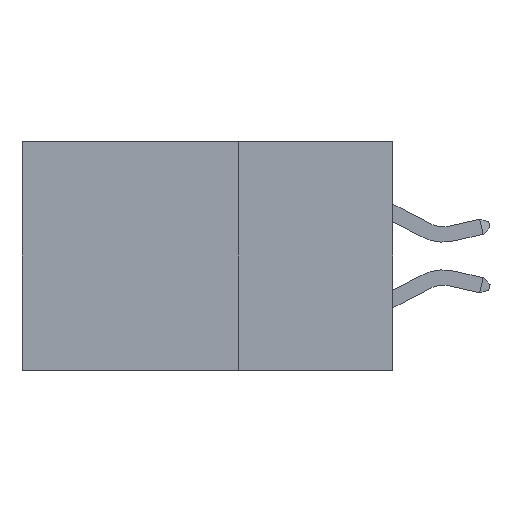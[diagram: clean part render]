
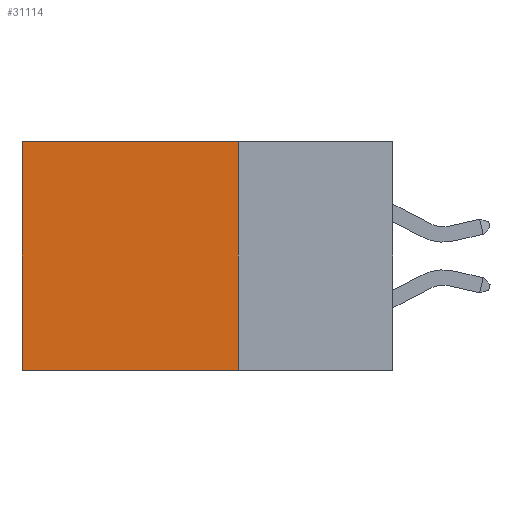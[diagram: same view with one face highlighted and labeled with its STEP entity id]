
A CAD part, left-side view. The second image highlights one B-rep face of the part: STEP entity #31114.
In plain terms, the highlighted planar face has unit normal (-1, 0, 0).
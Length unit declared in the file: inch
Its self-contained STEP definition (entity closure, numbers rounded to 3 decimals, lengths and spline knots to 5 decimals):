
#71 = LINE ( 'NONE', #34770, #13173 ) ;
#74 = CARTESIAN_POINT ( 'NONE',  ( 0.2875, 0.25, -0.37 ) ) ;
#258 = AXIS2_PLACEMENT_3D ( 'NONE', #278, #2641, #8161 ) ;
#278 = CARTESIAN_POINT ( 'NONE',  ( 0.2875, 0.25, 0. ) ) ;
#772 = CARTESIAN_POINT ( 'NONE',  ( 0.2875, 0.6, 0. ) ) ;
#2343 = CARTESIAN_POINT ( 'NONE',  ( 0.2875, 0.25, 0. ) ) ;
#2641 = DIRECTION ( 'NONE',  ( 1., 0., 0. ) ) ;
#3703 = ORIENTED_EDGE ( 'NONE', *, *, #32544, .F. ) ;
#3853 = EDGE_CURVE ( 'NONE', #13371, #12903, #31158, .T. ) ;
#4574 = DIRECTION ( 'NONE',  ( 0., 1., 0. ) ) ;
#4733 = FACE_OUTER_BOUND ( 'NONE', #22316, .T. ) ;
#5043 = LINE ( 'NONE', #17857, #17332 ) ;
#5070 = VECTOR ( 'NONE', #13770, 39.37008 ) ;
#7614 = VERTEX_POINT ( 'NONE', #25218 ) ;
#8161 = DIRECTION ( 'NONE',  ( 0., 0., -1. ) ) ;
#10586 = EDGE_CURVE ( 'NONE', #13371, #14467, #5043, .T. ) ;
#12903 = VERTEX_POINT ( 'NONE', #19934 ) ;
#13173 = VECTOR ( 'NONE', #33191, 39.37008 ) ;
#13371 = VERTEX_POINT ( 'NONE', #33732 ) ;
#13546 = DIRECTION ( 'NONE',  ( 0., 0., -1. ) ) ;
#13610 = ORIENTED_EDGE ( 'NONE', *, *, #18839, .T. ) ;
#13770 = DIRECTION ( 'NONE',  ( 0., 1., 0. ) ) ;
#14467 = VERTEX_POINT ( 'NONE', #772 ) ;
#15407 = ORIENTED_EDGE ( 'NONE', *, *, #10586, .T. ) ;
#16140 = PLANE ( 'NONE',  #258 ) ;
#17332 = VECTOR ( 'NONE', #4574, 39.37008 ) ;
#17857 = CARTESIAN_POINT ( 'NONE',  ( 0.2875, 0.25, 0. ) ) ;
#18105 = ORIENTED_EDGE ( 'NONE', *, *, #3853, .F. ) ;
#18839 = EDGE_CURVE ( 'NONE', #14467, #7614, #71, .T. ) ;
#19503 = LINE ( 'NONE', #74, #5070 ) ;
#19934 = CARTESIAN_POINT ( 'NONE',  ( 0.2875, 0.25, -0.37 ) ) ;
#22316 = EDGE_LOOP ( 'NONE', ( #13610, #3703, #18105, #15407 ) ) ;
#25218 = CARTESIAN_POINT ( 'NONE',  ( 0.2875, 0.6, -0.37 ) ) ;
#26887 = VECTOR ( 'NONE', #13546, 39.37008 ) ;
#31114 = ADVANCED_FACE ( 'NONE', ( #4733 ), #16140, .F. ) ;
#31158 = LINE ( 'NONE', #2343, #26887 ) ;
#32544 = EDGE_CURVE ( 'NONE', #12903, #7614, #19503, .T. ) ;
#33191 = DIRECTION ( 'NONE',  ( 0., 0., -1. ) ) ;
#33732 = CARTESIAN_POINT ( 'NONE',  ( 0.2875, 0.25, 0. ) ) ;
#34770 = CARTESIAN_POINT ( 'NONE',  ( 0.2875, 0.6, 0. ) ) ;
